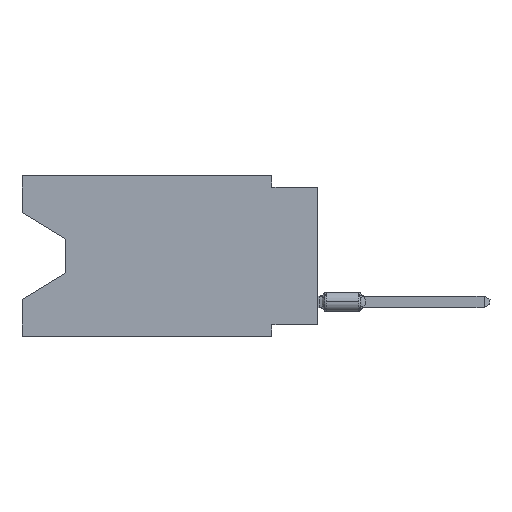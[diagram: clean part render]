
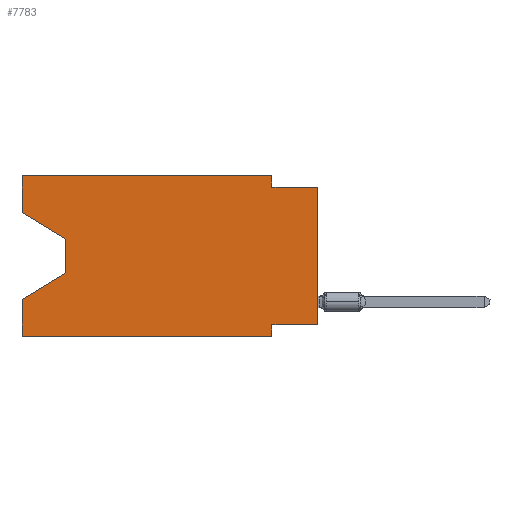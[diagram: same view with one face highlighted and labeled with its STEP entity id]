
A CAD part, left-side view. The second image highlights one B-rep face of the part: STEP entity #7783.
In plain terms, the highlighted planar face has unit normal (-1, 0, 0).
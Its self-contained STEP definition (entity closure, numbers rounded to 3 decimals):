
#81 = CARTESIAN_POINT ( 'NONE',  ( 0., 16.383, 0. ) ) ;
#276 = VERTEX_POINT ( 'NONE', #12264 ) ;
#316 = LINE ( 'NONE', #20421, #2416 ) ;
#405 = CARTESIAN_POINT ( 'NONE',  ( 0., 13.97, -3.505 ) ) ;
#818 = VERTEX_POINT ( 'NONE', #10190 ) ;
#1153 = CARTESIAN_POINT ( 'NONE',  ( 0., 13.97, -5.385 ) ) ;
#1163 = VERTEX_POINT ( 'NONE', #22595 ) ;
#1241 = CARTESIAN_POINT ( 'NONE',  ( 0., 16.383, -2.038 ) ) ;
#1326 = ORIENTED_EDGE ( 'NONE', *, *, #19065, .T. ) ;
#1995 = ORIENTED_EDGE ( 'NONE', *, *, #14938, .F. ) ;
#2008 = ORIENTED_EDGE ( 'NONE', *, *, #13146, .F. ) ;
#2416 = VECTOR ( 'NONE', #26567, 1000. ) ;
#3067 = VERTEX_POINT ( 'NONE', #5861 ) ;
#3287 = CARTESIAN_POINT ( 'NONE',  ( 0., 13.97, -5.385 ) ) ;
#3309 = CARTESIAN_POINT ( 'NONE',  ( 0., 2.54, -8.89 ) ) ;
#3501 = EDGE_CURVE ( 'NONE', #1163, #22064, #18983, .T. ) ;
#3644 = CARTESIAN_POINT ( 'NONE',  ( 0., 0., 0. ) ) ;
#3703 = VECTOR ( 'NONE', #8510, 1000. ) ;
#4068 = DIRECTION ( 'NONE',  ( 0., 0., 1. ) ) ;
#4351 = VECTOR ( 'NONE', #25827, 1000. ) ;
#4386 = EDGE_CURVE ( 'NONE', #15722, #21862, #6120, .T. ) ;
#4666 = VERTEX_POINT ( 'NONE', #24398 ) ;
#4889 = VECTOR ( 'NONE', #25370, 1000. ) ;
#5019 = EDGE_CURVE ( 'NONE', #276, #22064, #16216, .T. ) ;
#5558 = LINE ( 'NONE', #19751, #21542 ) ;
#5843 = ORIENTED_EDGE ( 'NONE', *, *, #3501, .T. ) ;
#5861 = CARTESIAN_POINT ( 'NONE',  ( 0., 2.54, 0. ) ) ;
#5902 = CARTESIAN_POINT ( 'NONE',  ( 0., 16.383, -6.852 ) ) ;
#5941 = DIRECTION ( 'NONE',  ( 0., 0., 1. ) ) ;
#6120 = LINE ( 'NONE', #14436, #12027 ) ;
#6735 = VERTEX_POINT ( 'NONE', #1153 ) ;
#7152 = FACE_OUTER_BOUND ( 'NONE', #19326, .T. ) ;
#7460 = DIRECTION ( 'NONE',  ( 0., -0.855, -0.519 ) ) ;
#7505 = DIRECTION ( 'NONE',  ( 0., 0., -1. ) ) ;
#7783 = ADVANCED_FACE ( 'NONE', ( #7152 ), #13830, .F. ) ;
#8510 = DIRECTION ( 'NONE',  ( 0., -1., 0. ) ) ;
#8627 = EDGE_CURVE ( 'NONE', #15722, #14430, #26169, .T. ) ;
#8901 = VECTOR ( 'NONE', #18262, 1000. ) ;
#9358 = ORIENTED_EDGE ( 'NONE', *, *, #8627, .T. ) ;
#9610 = EDGE_CURVE ( 'NONE', #1163, #22010, #18364, .T. ) ;
#9685 = AXIS2_PLACEMENT_3D ( 'NONE', #17657, #25854, #26764 ) ;
#9970 = CARTESIAN_POINT ( 'NONE',  ( 0., 2.54, 0. ) ) ;
#10190 = CARTESIAN_POINT ( 'NONE',  ( 0., 2.54, -0.635 ) ) ;
#10219 = EDGE_CURVE ( 'NONE', #6735, #22010, #11617, .T. ) ;
#10343 = ORIENTED_EDGE ( 'NONE', *, *, #5019, .F. ) ;
#10895 = LINE ( 'NONE', #405, #4889 ) ;
#11149 = ORIENTED_EDGE ( 'NONE', *, *, #12857, .T. ) ;
#11617 = LINE ( 'NONE', #3287, #4351 ) ;
#12027 = VECTOR ( 'NONE', #4068, 1000. ) ;
#12075 = LINE ( 'NONE', #25036, #3703 ) ;
#12132 = VECTOR ( 'NONE', #16829, 1000. ) ;
#12264 = CARTESIAN_POINT ( 'NONE',  ( 0., 2.54, -8.255 ) ) ;
#12269 = VECTOR ( 'NONE', #7460, 1000. ) ;
#12471 = VECTOR ( 'NONE', #7505, 1000. ) ;
#12857 = EDGE_CURVE ( 'NONE', #4666, #15736, #22362, .T. ) ;
#13146 = EDGE_CURVE ( 'NONE', #818, #15736, #5558, .T. ) ;
#13400 = ORIENTED_EDGE ( 'NONE', *, *, #4386, .F. ) ;
#13830 = PLANE ( 'NONE',  #9685 ) ;
#14430 = VERTEX_POINT ( 'NONE', #24309 ) ;
#14436 = CARTESIAN_POINT ( 'NONE',  ( 0., 16.383, 0. ) ) ;
#14938 = EDGE_CURVE ( 'NONE', #21862, #3067, #12075, .T. ) ;
#15187 = CARTESIAN_POINT ( 'NONE',  ( 0., 16.383, 0. ) ) ;
#15234 = VECTOR ( 'NONE', #5941, 1000. ) ;
#15722 = VERTEX_POINT ( 'NONE', #1241 ) ;
#15736 = VERTEX_POINT ( 'NONE', #15829 ) ;
#15829 = CARTESIAN_POINT ( 'NONE',  ( 0., 0., -0.635 ) ) ;
#16216 = LINE ( 'NONE', #26869, #20781 ) ;
#16348 = DIRECTION ( 'NONE',  ( 0., 0., -1. ) ) ;
#16385 = ORIENTED_EDGE ( 'NONE', *, *, #9610, .F. ) ;
#16747 = ORIENTED_EDGE ( 'NONE', *, *, #17585, .F. ) ;
#16829 = DIRECTION ( 'NONE',  ( 0., -1., 0. ) ) ;
#16940 = CARTESIAN_POINT ( 'NONE',  ( 0., 16.383, -8.89 ) ) ;
#17585 = EDGE_CURVE ( 'NONE', #3067, #818, #26211, .T. ) ;
#17657 = CARTESIAN_POINT ( 'NONE',  ( 0., 16.383, 0. ) ) ;
#18262 = DIRECTION ( 'NONE',  ( 0., 0., 1. ) ) ;
#18364 = LINE ( 'NONE', #81, #15234 ) ;
#18983 = LINE ( 'NONE', #16940, #12132 ) ;
#19065 = EDGE_CURVE ( 'NONE', #14430, #6735, #10895, .T. ) ;
#19326 = EDGE_LOOP ( 'NONE', ( #9358, #1326, #19925, #16385, #5843, #10343, #25080, #11149, #2008, #16747, #1995, #13400 ) ) ;
#19751 = CARTESIAN_POINT ( 'NONE',  ( 0., 0., -0.635 ) ) ;
#19925 = ORIENTED_EDGE ( 'NONE', *, *, #10219, .T. ) ;
#20012 = CARTESIAN_POINT ( 'NONE',  ( 0., 16.383, -2.038 ) ) ;
#20421 = CARTESIAN_POINT ( 'NONE',  ( 0., 0., -8.255 ) ) ;
#20781 = VECTOR ( 'NONE', #16348, 1000. ) ;
#21542 = VECTOR ( 'NONE', #26176, 1000. ) ;
#21862 = VERTEX_POINT ( 'NONE', #15187 ) ;
#22010 = VERTEX_POINT ( 'NONE', #5902 ) ;
#22064 = VERTEX_POINT ( 'NONE', #3309 ) ;
#22362 = LINE ( 'NONE', #3644, #8901 ) ;
#22595 = CARTESIAN_POINT ( 'NONE',  ( 0., 16.383, -8.89 ) ) ;
#23366 = EDGE_CURVE ( 'NONE', #4666, #276, #316, .T. ) ;
#24309 = CARTESIAN_POINT ( 'NONE',  ( 0., 13.97, -3.505 ) ) ;
#24398 = CARTESIAN_POINT ( 'NONE',  ( 0., 0., -8.255 ) ) ;
#25036 = CARTESIAN_POINT ( 'NONE',  ( 0., 16.383, 0. ) ) ;
#25080 = ORIENTED_EDGE ( 'NONE', *, *, #23366, .F. ) ;
#25370 = DIRECTION ( 'NONE',  ( 0., 0., -1. ) ) ;
#25827 = DIRECTION ( 'NONE',  ( 0., 0.855, -0.519 ) ) ;
#25854 = DIRECTION ( 'NONE',  ( 1., 0., 0. ) ) ;
#26169 = LINE ( 'NONE', #20012, #12269 ) ;
#26176 = DIRECTION ( 'NONE',  ( 0., -1., 0. ) ) ;
#26211 = LINE ( 'NONE', #9970, #12471 ) ;
#26567 = DIRECTION ( 'NONE',  ( 0., 1., 0. ) ) ;
#26764 = DIRECTION ( 'NONE',  ( 0., 0., -1. ) ) ;
#26869 = CARTESIAN_POINT ( 'NONE',  ( 0., 2.54, -8.89 ) ) ;
